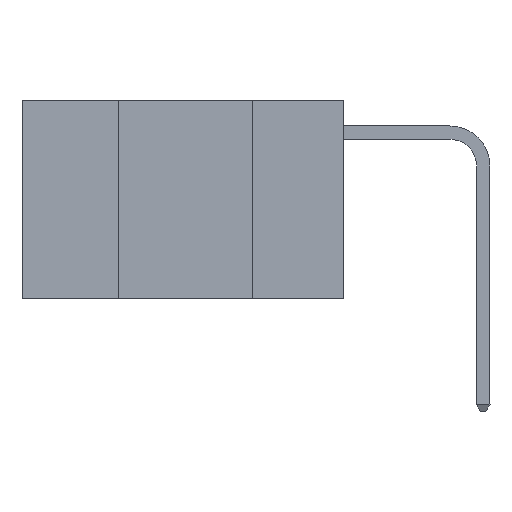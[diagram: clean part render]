
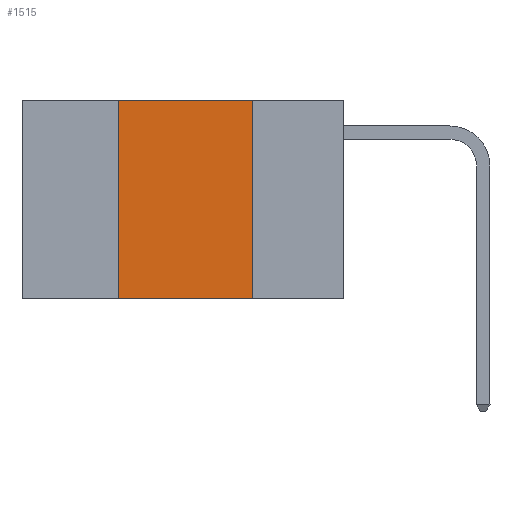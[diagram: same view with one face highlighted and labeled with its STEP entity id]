
A CAD part, left-side view. The second image highlights one B-rep face of the part: STEP entity #1515.
In plain terms, the highlighted planar face has unit normal (-1, 0, 0).
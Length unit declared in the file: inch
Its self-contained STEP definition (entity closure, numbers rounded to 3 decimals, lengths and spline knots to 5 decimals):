
#87 = LINE ( 'NONE', #7057, #1895 ) ;
#763 = LINE ( 'NONE', #12965, #16739 ) ;
#1515 = ADVANCED_FACE ( 'NONE', ( #18548 ), #9724, .F. ) ;
#1895 = VECTOR ( 'NONE', #7298, 39.37008 ) ;
#2324 = DIRECTION ( 'NONE',  ( 1., 0., 0. ) ) ;
#2777 = ORIENTED_EDGE ( 'NONE', *, *, #8959, .F. ) ;
#2851 = VECTOR ( 'NONE', #10761, 39.37008 ) ;
#3056 = VECTOR ( 'NONE', #10214, 39.37008 ) ;
#3303 = CARTESIAN_POINT ( 'NONE',  ( 0., 0.42, -0.37 ) ) ;
#3351 = CARTESIAN_POINT ( 'NONE',  ( 0., 0.17, 0. ) ) ;
#3363 = VERTEX_POINT ( 'NONE', #3303 ) ;
#3776 = ORIENTED_EDGE ( 'NONE', *, *, #6517, .F. ) ;
#3997 = DIRECTION ( 'NONE',  ( 0., 0., 1. ) ) ;
#5648 = EDGE_CURVE ( 'NONE', #3363, #15315, #87, .T. ) ;
#6517 = EDGE_CURVE ( 'NONE', #3363, #13768, #763, .T. ) ;
#7057 = CARTESIAN_POINT ( 'NONE',  ( 0., 0.6, -0.37 ) ) ;
#7298 = DIRECTION ( 'NONE',  ( 0., -1., 0. ) ) ;
#8959 = EDGE_CURVE ( 'NONE', #21257, #15315, #16660, .T. ) ;
#9637 = CARTESIAN_POINT ( 'NONE',  ( 0., 0.17, 0. ) ) ;
#9724 = PLANE ( 'NONE',  #20605 ) ;
#9947 = CARTESIAN_POINT ( 'NONE',  ( 0., 0.6, 0. ) ) ;
#10214 = DIRECTION ( 'NONE',  ( 0., -1., 0. ) ) ;
#10761 = DIRECTION ( 'NONE',  ( 0., 0., -1. ) ) ;
#12005 = LINE ( 'NONE', #17582, #3056 ) ;
#12965 = CARTESIAN_POINT ( 'NONE',  ( 0., 0.42, 0. ) ) ;
#13419 = DIRECTION ( 'NONE',  ( 0., 0., -1. ) ) ;
#13602 = CARTESIAN_POINT ( 'NONE',  ( 0., 0.42, 0. ) ) ;
#13768 = VERTEX_POINT ( 'NONE', #13602 ) ;
#13815 = CARTESIAN_POINT ( 'NONE',  ( 0., 0.17, -0.37 ) ) ;
#15315 = VERTEX_POINT ( 'NONE', #13815 ) ;
#15520 = ORIENTED_EDGE ( 'NONE', *, *, #5648, .T. ) ;
#16660 = LINE ( 'NONE', #9637, #2851 ) ;
#16739 = VECTOR ( 'NONE', #3997, 39.37008 ) ;
#17582 = CARTESIAN_POINT ( 'NONE',  ( 0., 0.6, 0. ) ) ;
#18548 = FACE_OUTER_BOUND ( 'NONE', #22100, .T. ) ;
#19920 = EDGE_CURVE ( 'NONE', #13768, #21257, #12005, .T. ) ;
#20605 = AXIS2_PLACEMENT_3D ( 'NONE', #9947, #2324, #13419 ) ;
#21257 = VERTEX_POINT ( 'NONE', #3351 ) ;
#21686 = ORIENTED_EDGE ( 'NONE', *, *, #19920, .F. ) ;
#22100 = EDGE_LOOP ( 'NONE', ( #2777, #21686, #3776, #15520 ) ) ;
